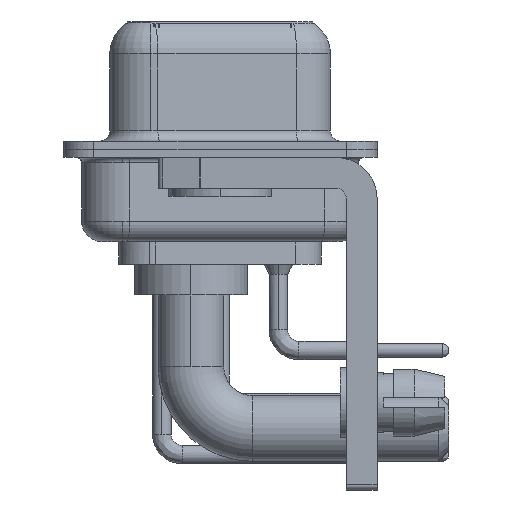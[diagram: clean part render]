
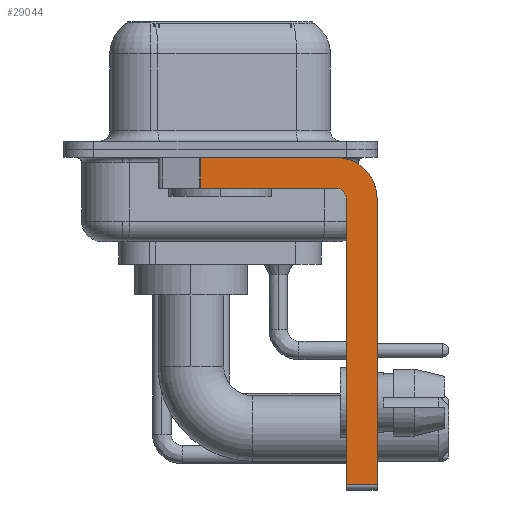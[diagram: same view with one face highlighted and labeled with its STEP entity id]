
A CAD part, left-side view. The second image highlights one B-rep face of the part: STEP entity #29044.
In plain terms, the highlighted planar face has unit normal (-1, 0, 0).
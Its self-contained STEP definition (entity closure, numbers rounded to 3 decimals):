
#60 = EDGE_CURVE ( 'NONE', #27135, #28935, #34961, .T. ) ;
#1013 = CARTESIAN_POINT ( 'NONE',  ( -2.9, 0.978, -1.9 ) ) ;
#1198 = AXIS2_PLACEMENT_3D ( 'NONE', #18440, #29670, #4436 ) ;
#1597 = EDGE_CURVE ( 'NONE', #7542, #27106, #30531, .T. ) ;
#1761 = CARTESIAN_POINT ( 'NONE',  ( -2.9, -5.65, -2.4 ) ) ;
#2091 = VECTOR ( 'NONE', #15475, 1000. ) ;
#2153 = CIRCLE ( 'NONE', #30362, 2. ) ;
#2329 = ORIENTED_EDGE ( 'NONE', *, *, #13522, .F. ) ;
#2377 = ORIENTED_EDGE ( 'NONE', *, *, #9166, .T. ) ;
#2622 = DIRECTION ( 'NONE',  ( -1., 0., 0. ) ) ;
#2825 = CARTESIAN_POINT ( 'NONE',  ( -2.9, 3., -0.4 ) ) ;
#3733 = VECTOR ( 'NONE', #26059, 1000. ) ;
#4436 = DIRECTION ( 'NONE',  ( 0., 0., -1. ) ) ;
#4834 = DIRECTION ( 'NONE',  ( 0., 0., -1. ) ) ;
#4915 = CIRCLE ( 'NONE', #35460, 0.5 ) ;
#5759 = VERTEX_POINT ( 'NONE', #6645 ) ;
#5887 = VECTOR ( 'NONE', #22695, 1000. ) ;
#6164 = CARTESIAN_POINT ( 'NONE',  ( -2.9, 0.978, -1.9 ) ) ;
#6645 = CARTESIAN_POINT ( 'NONE',  ( -2.9, -7.65, -2.4 ) ) ;
#6656 = ORIENTED_EDGE ( 'NONE', *, *, #27465, .F. ) ;
#7516 = CARTESIAN_POINT ( 'NONE',  ( -2.9, -5.65, -1.9 ) ) ;
#7542 = VERTEX_POINT ( 'NONE', #21108 ) ;
#7709 = VERTEX_POINT ( 'NONE', #14794 ) ;
#9166 = EDGE_CURVE ( 'NONE', #18984, #27106, #34508, .T. ) ;
#9371 = CARTESIAN_POINT ( 'NONE',  ( -2.9, -5.65, -16.35 ) ) ;
#10118 = CARTESIAN_POINT ( 'NONE',  ( -2.9, -6.15, -16.6 ) ) ;
#10544 = ORIENTED_EDGE ( 'NONE', *, *, #25010, .F. ) ;
#11472 = LINE ( 'NONE', #2825, #5887 ) ;
#12147 = DIRECTION ( 'NONE',  ( 0., -1., 0. ) ) ;
#12522 = LINE ( 'NONE', #10118, #2091 ) ;
#12772 = VECTOR ( 'NONE', #4834, 1000. ) ;
#13299 = ORIENTED_EDGE ( 'NONE', *, *, #22052, .F. ) ;
#13522 = EDGE_CURVE ( 'NONE', #17790, #5759, #2153, .T. ) ;
#14794 = CARTESIAN_POINT ( 'NONE',  ( -2.9, -6.15, -2.4 ) ) ;
#15475 = DIRECTION ( 'NONE',  ( 0., 0., 1. ) ) ;
#16058 = DIRECTION ( 'NONE',  ( 0., 0., 1. ) ) ;
#16526 = CARTESIAN_POINT ( 'NONE',  ( -2.9, -5.65, -0.4 ) ) ;
#17374 = ORIENTED_EDGE ( 'NONE', *, *, #60, .T. ) ;
#17555 = CARTESIAN_POINT ( 'NONE',  ( -2.9, -7.65, -2.4 ) ) ;
#17790 = VERTEX_POINT ( 'NONE', #16526 ) ;
#18440 = CARTESIAN_POINT ( 'NONE',  ( -2.9, -5.65, -2.4 ) ) ;
#18683 = DIRECTION ( 'NONE',  ( 1., 0., 0. ) ) ;
#18806 = CARTESIAN_POINT ( 'NONE',  ( -2.9, -5.65, -2.4 ) ) ;
#18984 = VERTEX_POINT ( 'NONE', #32717 ) ;
#20479 = EDGE_CURVE ( 'NONE', #7709, #7542, #4915, .T. ) ;
#21108 = CARTESIAN_POINT ( 'NONE',  ( -2.9, -5.65, -1.9 ) ) ;
#21684 = ORIENTED_EDGE ( 'NONE', *, *, #20479, .F. ) ;
#21993 = DIRECTION ( 'NONE',  ( 0., 0., -1. ) ) ;
#22052 = EDGE_CURVE ( 'NONE', #27135, #7709, #12522, .T. ) ;
#22695 = DIRECTION ( 'NONE',  ( 0., -1., 0. ) ) ;
#23975 = FACE_OUTER_BOUND ( 'NONE', #33386, .T. ) ;
#25010 = EDGE_CURVE ( 'NONE', #5759, #28935, #31547, .T. ) ;
#25017 = DIRECTION ( 'NONE',  ( 0., 1., 0. ) ) ;
#26059 = DIRECTION ( 'NONE',  ( 0., 0., -1. ) ) ;
#27106 = VERTEX_POINT ( 'NONE', #1013 ) ;
#27135 = VERTEX_POINT ( 'NONE', #34852 ) ;
#27465 = EDGE_CURVE ( 'NONE', #18984, #17790, #11472, .T. ) ;
#28935 = VERTEX_POINT ( 'NONE', #32601 ) ;
#29044 = ADVANCED_FACE ( 'NONE', ( #23975 ), #35182, .F. ) ;
#29613 = VECTOR ( 'NONE', #25017, 1000. ) ;
#29670 = DIRECTION ( 'NONE',  ( 1., 0., 0. ) ) ;
#30362 = AXIS2_PLACEMENT_3D ( 'NONE', #1761, #18683, #21993 ) ;
#30531 = LINE ( 'NONE', #7516, #29613 ) ;
#31547 = LINE ( 'NONE', #17555, #12772 ) ;
#31880 = VECTOR ( 'NONE', #12147, 1000. ) ;
#32601 = CARTESIAN_POINT ( 'NONE',  ( -2.9, -7.65, -16.35 ) ) ;
#32717 = CARTESIAN_POINT ( 'NONE',  ( -2.9, 0.978, -0.4 ) ) ;
#33386 = EDGE_LOOP ( 'NONE', ( #6656, #2377, #34717, #21684, #13299, #17374, #10544, #2329 ) ) ;
#34508 = LINE ( 'NONE', #6164, #3733 ) ;
#34717 = ORIENTED_EDGE ( 'NONE', *, *, #1597, .F. ) ;
#34852 = CARTESIAN_POINT ( 'NONE',  ( -2.9, -6.15, -16.35 ) ) ;
#34961 = LINE ( 'NONE', #9371, #31880 ) ;
#35182 = PLANE ( 'NONE',  #1198 ) ;
#35460 = AXIS2_PLACEMENT_3D ( 'NONE', #18806, #2622, #16058 ) ;
